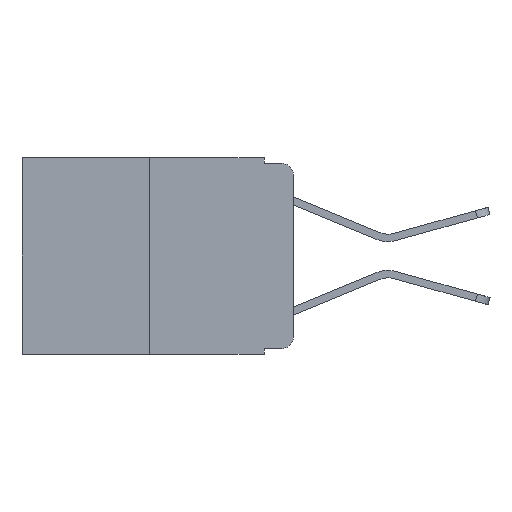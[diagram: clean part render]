
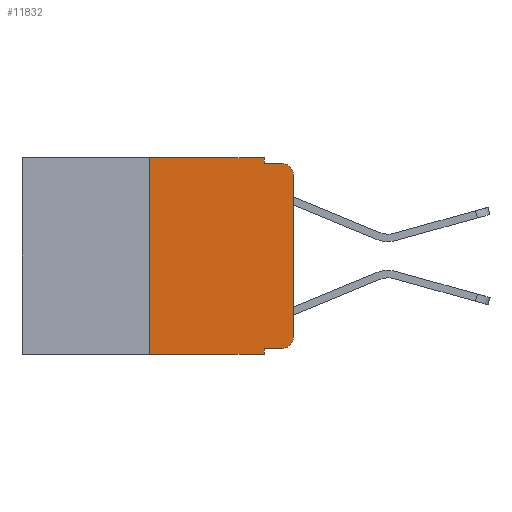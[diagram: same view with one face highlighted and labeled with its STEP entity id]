
A CAD part, left-side view. The second image highlights one B-rep face of the part: STEP entity #11832.
In plain terms, the highlighted planar face has unit normal (-1, 0, 0).
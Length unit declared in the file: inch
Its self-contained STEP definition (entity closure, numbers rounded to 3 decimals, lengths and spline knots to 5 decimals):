
#180 = VERTEX_POINT ( 'NONE', #15854 ) ;
#403 = VERTEX_POINT ( 'NONE', #8515 ) ;
#482 = EDGE_CURVE ( 'NONE', #10136, #5766, #14781, .T. ) ;
#696 = VERTEX_POINT ( 'NONE', #10412 ) ;
#704 = EDGE_CURVE ( 'NONE', #180, #17713, #2184, .T. ) ;
#717 = DIRECTION ( 'NONE',  ( 0., 0., 1. ) ) ;
#1010 = CARTESIAN_POINT ( 'NONE',  ( 0., 0.473, -0.343 ) ) ;
#1101 = ORIENTED_EDGE ( 'NONE', *, *, #15307, .T. ) ;
#1160 = LINE ( 'NONE', #4158, #16532 ) ;
#1227 = VECTOR ( 'NONE', #3814, 39.37008 ) ;
#1403 = VERTEX_POINT ( 'NONE', #16687 ) ;
#1477 = ORIENTED_EDGE ( 'NONE', *, *, #482, .T. ) ;
#1579 = CARTESIAN_POINT ( 'NONE',  ( 0., 0.051, 0. ) ) ;
#1759 = VECTOR ( 'NONE', #16787, 39.37008 ) ;
#1767 = ORIENTED_EDGE ( 'NONE', *, *, #3287, .F. ) ;
#1815 = AXIS2_PLACEMENT_3D ( 'NONE', #7610, #7424, #8908 ) ;
#2184 = LINE ( 'NONE', #1579, #1759 ) ;
#2498 = LINE ( 'NONE', #8842, #7539 ) ;
#2615 = ORIENTED_EDGE ( 'NONE', *, *, #704, .F. ) ;
#2740 = VERTEX_POINT ( 'NONE', #12847 ) ;
#2789 = DIRECTION ( 'NONE',  ( 0., 0., -1. ) ) ;
#2823 = DIRECTION ( 'NONE',  ( 0., 0., -1. ) ) ;
#2871 = FACE_OUTER_BOUND ( 'NONE', #4202, .T. ) ;
#2935 = CARTESIAN_POINT ( 'NONE',  ( 0., 0.02, -0.01 ) ) ;
#3287 = EDGE_CURVE ( 'NONE', #2740, #14885, #12761, .T. ) ;
#3564 = AXIS2_PLACEMENT_3D ( 'NONE', #15120, #8139, #5367 ) ;
#3814 = DIRECTION ( 'NONE',  ( 0., -1., 0. ) ) ;
#3868 = CARTESIAN_POINT ( 'NONE',  ( 0., 0.02, -0.333 ) ) ;
#3988 = PLANE ( 'NONE',  #3564 ) ;
#4158 = CARTESIAN_POINT ( 'NONE',  ( 0., 0.473, 0. ) ) ;
#4202 = EDGE_LOOP ( 'NONE', ( #1101, #17322, #17864, #1767, #17706, #12691, #8777, #2615, #12947, #1477 ) ) ;
#4969 = CARTESIAN_POINT ( 'NONE',  ( 0., 0.051, -0.01 ) ) ;
#5138 = CARTESIAN_POINT ( 'NONE',  ( 0., 0.051, -0.333 ) ) ;
#5367 = DIRECTION ( 'NONE',  ( 0., 0., -1. ) ) ;
#5766 = VERTEX_POINT ( 'NONE', #6940 ) ;
#6377 = VECTOR ( 'NONE', #15303, 39.37008 ) ;
#6940 = CARTESIAN_POINT ( 'NONE',  ( 0., 0., -0.313 ) ) ;
#7424 = DIRECTION ( 'NONE',  ( -1., 0., 0. ) ) ;
#7539 = VECTOR ( 'NONE', #717, 39.37008 ) ;
#7610 = CARTESIAN_POINT ( 'NONE',  ( 0., 0.02, -0.03 ) ) ;
#7648 = CIRCLE ( 'NONE', #1815, 0.02 ) ;
#8072 = EDGE_CURVE ( 'NONE', #14885, #11961, #17413, .T. ) ;
#8139 = DIRECTION ( 'NONE',  ( 1., 0., 0. ) ) ;
#8402 = EDGE_CURVE ( 'NONE', #696, #17713, #14337, .T. ) ;
#8515 = CARTESIAN_POINT ( 'NONE',  ( 0., 0.25, 0. ) ) ;
#8557 = DIRECTION ( 'NONE',  ( 0., -1., 0. ) ) ;
#8777 = ORIENTED_EDGE ( 'NONE', *, *, #8402, .T. ) ;
#8842 = CARTESIAN_POINT ( 'NONE',  ( 0., 0.25, 0. ) ) ;
#8908 = DIRECTION ( 'NONE',  ( 0., 0., -1. ) ) ;
#9439 = EDGE_CURVE ( 'NONE', #696, #403, #2498, .T. ) ;
#9487 = LINE ( 'NONE', #9762, #6377 ) ;
#9762 = CARTESIAN_POINT ( 'NONE',  ( 0., 0., 0. ) ) ;
#10136 = VERTEX_POINT ( 'NONE', #3868 ) ;
#10412 = CARTESIAN_POINT ( 'NONE',  ( 0., 0.25, -0.343 ) ) ;
#10594 = DIRECTION ( 'NONE',  ( 0., -1., 0. ) ) ;
#10649 = CARTESIAN_POINT ( 'NONE',  ( 0., 0.051, -0.343 ) ) ;
#11151 = CARTESIAN_POINT ( 'NONE',  ( 0., 0.051, 0. ) ) ;
#11183 = CARTESIAN_POINT ( 'NONE',  ( 0., 0.02, -0.313 ) ) ;
#11328 = VECTOR ( 'NONE', #10594, 39.37008 ) ;
#11832 = ADVANCED_FACE ( 'NONE', ( #2871 ), #3988, .F. ) ;
#11961 = VERTEX_POINT ( 'NONE', #2935 ) ;
#12691 = ORIENTED_EDGE ( 'NONE', *, *, #9439, .F. ) ;
#12761 = LINE ( 'NONE', #11151, #17334 ) ;
#12762 = EDGE_CURVE ( 'NONE', #1403, #11961, #7648, .T. ) ;
#12847 = CARTESIAN_POINT ( 'NONE',  ( 0., 0.051, 0. ) ) ;
#12947 = ORIENTED_EDGE ( 'NONE', *, *, #15035, .T. ) ;
#12997 = CARTESIAN_POINT ( 'NONE',  ( 0., 0.051, -0.01 ) ) ;
#13712 = VECTOR ( 'NONE', #14528, 39.37008 ) ;
#14337 = LINE ( 'NONE', #1010, #11328 ) ;
#14528 = DIRECTION ( 'NONE',  ( 0., -1., 0. ) ) ;
#14677 = LINE ( 'NONE', #5138, #1227 ) ;
#14781 = CIRCLE ( 'NONE', #16983, 0.02 ) ;
#14885 = VERTEX_POINT ( 'NONE', #12997 ) ;
#15035 = EDGE_CURVE ( 'NONE', #180, #10136, #14677, .T. ) ;
#15120 = CARTESIAN_POINT ( 'NONE',  ( 0., 0.473, 0. ) ) ;
#15277 = EDGE_CURVE ( 'NONE', #403, #2740, #1160, .T. ) ;
#15303 = DIRECTION ( 'NONE',  ( 0., 0., 1. ) ) ;
#15307 = EDGE_CURVE ( 'NONE', #5766, #1403, #9487, .T. ) ;
#15854 = CARTESIAN_POINT ( 'NONE',  ( 0., 0.051, -0.333 ) ) ;
#16532 = VECTOR ( 'NONE', #8557, 39.37008 ) ;
#16687 = CARTESIAN_POINT ( 'NONE',  ( 0., 0., -0.03 ) ) ;
#16787 = DIRECTION ( 'NONE',  ( 0., 0., -1. ) ) ;
#16983 = AXIS2_PLACEMENT_3D ( 'NONE', #11183, #17906, #2789 ) ;
#17322 = ORIENTED_EDGE ( 'NONE', *, *, #12762, .T. ) ;
#17334 = VECTOR ( 'NONE', #2823, 39.37008 ) ;
#17413 = LINE ( 'NONE', #4969, #13712 ) ;
#17706 = ORIENTED_EDGE ( 'NONE', *, *, #15277, .F. ) ;
#17713 = VERTEX_POINT ( 'NONE', #10649 ) ;
#17864 = ORIENTED_EDGE ( 'NONE', *, *, #8072, .F. ) ;
#17906 = DIRECTION ( 'NONE',  ( -1., 0., 0. ) ) ;
